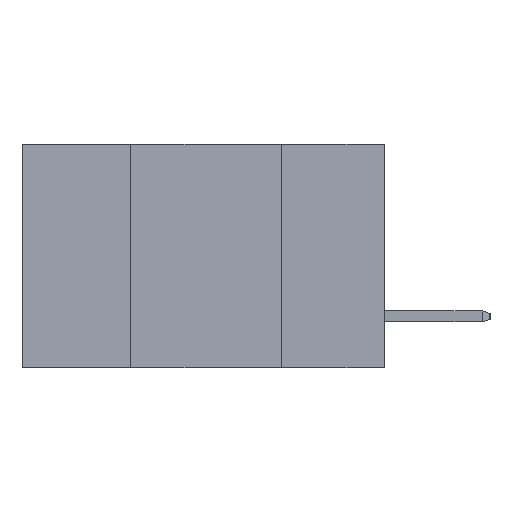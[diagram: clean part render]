
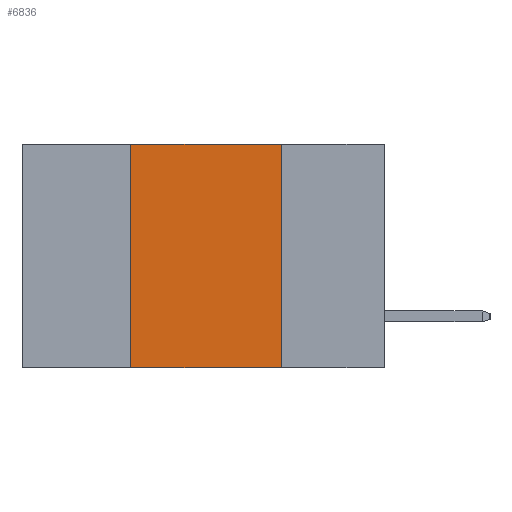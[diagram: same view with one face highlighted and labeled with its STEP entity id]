
A CAD part, left-side view. The second image highlights one B-rep face of the part: STEP entity #6836.
In plain terms, the highlighted planar face has unit normal (-1, 0, 0).
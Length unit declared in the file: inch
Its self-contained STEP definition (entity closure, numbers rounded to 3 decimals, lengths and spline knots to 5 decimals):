
#665 = VERTEX_POINT ( 'NONE', #10677 ) ;
#1138 = FACE_OUTER_BOUND ( 'NONE', #10937, .T. ) ;
#1727 = AXIS2_PLACEMENT_3D ( 'NONE', #6982, #6426, #6392 ) ;
#2053 = ORIENTED_EDGE ( 'NONE', *, *, #12347, .T. ) ;
#3122 = VECTOR ( 'NONE', #18845, 39.37008 ) ;
#5549 = LINE ( 'NONE', #6748, #14130 ) ;
#6392 = DIRECTION ( 'NONE',  ( 0., 0., -1. ) ) ;
#6426 = DIRECTION ( 'NONE',  ( 1., 0., 0. ) ) ;
#6567 = PLANE ( 'NONE',  #1727 ) ;
#6748 = CARTESIAN_POINT ( 'NONE',  ( 0., 0.6, -0.37 ) ) ;
#6836 = ADVANCED_FACE ( 'NONE', ( #1138 ), #6567, .F. ) ;
#6982 = CARTESIAN_POINT ( 'NONE',  ( 0., 0.6, 0. ) ) ;
#7029 = LINE ( 'NONE', #14175, #14610 ) ;
#7243 = EDGE_CURVE ( 'NONE', #15117, #13898, #18639, .T. ) ;
#8440 = CARTESIAN_POINT ( 'NONE',  ( 0., 0.17, 0. ) ) ;
#9325 = EDGE_CURVE ( 'NONE', #10822, #15117, #7029, .T. ) ;
#10677 = CARTESIAN_POINT ( 'NONE',  ( 0., 0.17, -0.37 ) ) ;
#10822 = VERTEX_POINT ( 'NONE', #13721 ) ;
#10937 = EDGE_LOOP ( 'NONE', ( #14778, #18513, #13877, #2053 ) ) ;
#12347 = EDGE_CURVE ( 'NONE', #10822, #665, #5549, .T. ) ;
#13721 = CARTESIAN_POINT ( 'NONE',  ( 0., 0.42, -0.37 ) ) ;
#13877 = ORIENTED_EDGE ( 'NONE', *, *, #9325, .F. ) ;
#13898 = VERTEX_POINT ( 'NONE', #8440 ) ;
#14130 = VECTOR ( 'NONE', #15740, 39.37008 ) ;
#14175 = CARTESIAN_POINT ( 'NONE',  ( 0., 0.42, -0.37 ) ) ;
#14610 = VECTOR ( 'NONE', #15422, 39.37008 ) ;
#14778 = ORIENTED_EDGE ( 'NONE', *, *, #18463, .F. ) ;
#15117 = VERTEX_POINT ( 'NONE', #18428 ) ;
#15422 = DIRECTION ( 'NONE',  ( 0., 0., 1. ) ) ;
#15740 = DIRECTION ( 'NONE',  ( 0., -1., 0. ) ) ;
#18428 = CARTESIAN_POINT ( 'NONE',  ( 0., 0.42, 0. ) ) ;
#18463 = EDGE_CURVE ( 'NONE', #13898, #665, #18581, .T. ) ;
#18513 = ORIENTED_EDGE ( 'NONE', *, *, #7243, .F. ) ;
#18581 = LINE ( 'NONE', #18781, #3122 ) ;
#18639 = LINE ( 'NONE', #18959, #19064 ) ;
#18777 = DIRECTION ( 'NONE',  ( 0., -1., 0. ) ) ;
#18781 = CARTESIAN_POINT ( 'NONE',  ( 0., 0.17, -0.37 ) ) ;
#18845 = DIRECTION ( 'NONE',  ( 0., 0., -1. ) ) ;
#18959 = CARTESIAN_POINT ( 'NONE',  ( 0., 0.6, 0. ) ) ;
#19064 = VECTOR ( 'NONE', #18777, 39.37008 ) ;
